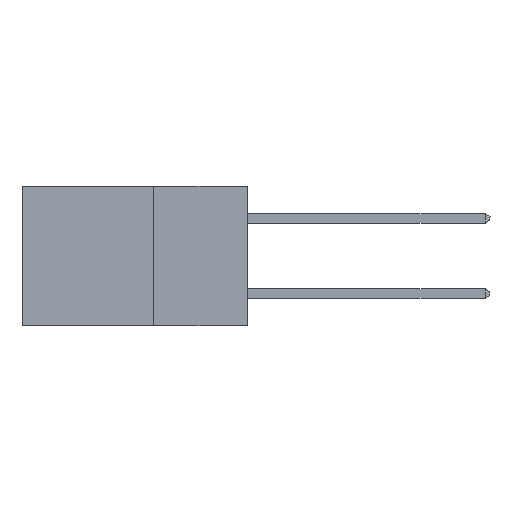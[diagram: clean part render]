
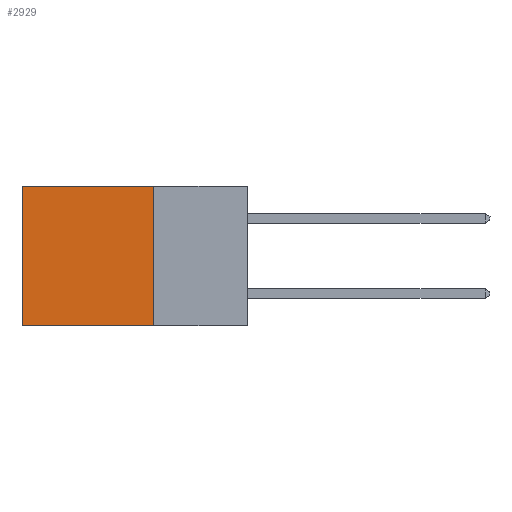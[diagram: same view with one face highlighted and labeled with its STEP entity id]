
A CAD part, left-side view. The second image highlights one B-rep face of the part: STEP entity #2929.
In plain terms, the highlighted planar face has unit normal (-1, 0, 0).
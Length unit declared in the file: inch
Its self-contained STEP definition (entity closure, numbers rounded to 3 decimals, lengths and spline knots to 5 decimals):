
#8 = CARTESIAN_POINT ( 'NONE',  ( 0.2615, 0.25, 0. ) ) ;
#698 = VERTEX_POINT ( 'NONE', #3398 ) ;
#1006 = DIRECTION ( 'NONE',  ( 0., 1., 0. ) ) ;
#1213 = DIRECTION ( 'NONE',  ( 0., 0., -1. ) ) ;
#1545 = ORIENTED_EDGE ( 'NONE', *, *, #6367, .F. ) ;
#1607 = DIRECTION ( 'NONE',  ( 0., 1., 0. ) ) ;
#1664 = LINE ( 'NONE', #8, #7726 ) ;
#1806 = CARTESIAN_POINT ( 'NONE',  ( 0.2615, 0.25, -0.37 ) ) ;
#2060 = DIRECTION ( 'NONE',  ( 0., 0., -1. ) ) ;
#2071 = CARTESIAN_POINT ( 'NONE',  ( 0.2615, 0.6, -0.37 ) ) ;
#2271 = VERTEX_POINT ( 'NONE', #1806 ) ;
#2929 = ADVANCED_FACE ( 'NONE', ( #5794 ), #5000, .F. ) ;
#3135 = VECTOR ( 'NONE', #11111, 39.37008 ) ;
#3398 = CARTESIAN_POINT ( 'NONE',  ( 0.2615, 0.6, -0.37 ) ) ;
#4851 = LINE ( 'NONE', #9234, #7138 ) ;
#4977 = CARTESIAN_POINT ( 'NONE',  ( 0.2615, 0.25, 0. ) ) ;
#5000 = PLANE ( 'NONE',  #6931 ) ;
#5794 = FACE_OUTER_BOUND ( 'NONE', #7798, .T. ) ;
#5815 = CARTESIAN_POINT ( 'NONE',  ( 0.2615, 0.25, -0.37 ) ) ;
#5851 = DIRECTION ( 'NONE',  ( 1., 0., 0. ) ) ;
#6367 = EDGE_CURVE ( 'NONE', #2271, #698, #4851, .T. ) ;
#6400 = ORIENTED_EDGE ( 'NONE', *, *, #10461, .F. ) ;
#6931 = AXIS2_PLACEMENT_3D ( 'NONE', #10620, #5851, #1213 ) ;
#7138 = VECTOR ( 'NONE', #1006, 39.37008 ) ;
#7436 = EDGE_CURVE ( 'NONE', #8132, #698, #7564, .T. ) ;
#7564 = LINE ( 'NONE', #2071, #3135 ) ;
#7726 = VECTOR ( 'NONE', #1607, 39.37008 ) ;
#7798 = EDGE_LOOP ( 'NONE', ( #10048, #1545, #6400, #11406 ) ) ;
#8132 = VERTEX_POINT ( 'NONE', #11735 ) ;
#8493 = LINE ( 'NONE', #5815, #8707 ) ;
#8655 = EDGE_CURVE ( 'NONE', #8910, #8132, #1664, .T. ) ;
#8707 = VECTOR ( 'NONE', #2060, 39.37008 ) ;
#8910 = VERTEX_POINT ( 'NONE', #4977 ) ;
#9234 = CARTESIAN_POINT ( 'NONE',  ( 0.2615, 0.25, -0.37 ) ) ;
#10048 = ORIENTED_EDGE ( 'NONE', *, *, #7436, .T. ) ;
#10461 = EDGE_CURVE ( 'NONE', #8910, #2271, #8493, .T. ) ;
#10620 = CARTESIAN_POINT ( 'NONE',  ( 0.2615, 0.25, -0.37 ) ) ;
#11111 = DIRECTION ( 'NONE',  ( 0., 0., -1. ) ) ;
#11406 = ORIENTED_EDGE ( 'NONE', *, *, #8655, .T. ) ;
#11735 = CARTESIAN_POINT ( 'NONE',  ( 0.2615, 0.6, 0. ) ) ;
